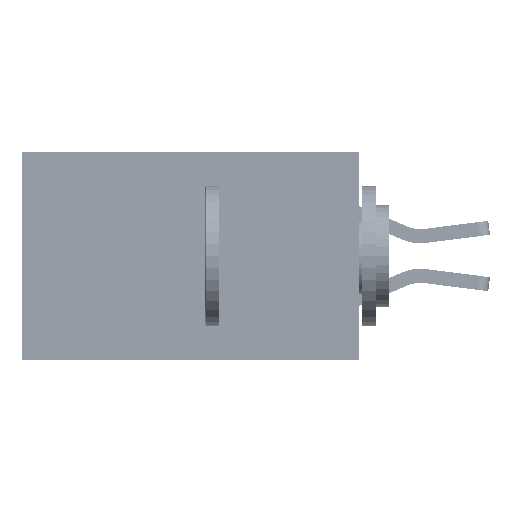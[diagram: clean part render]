
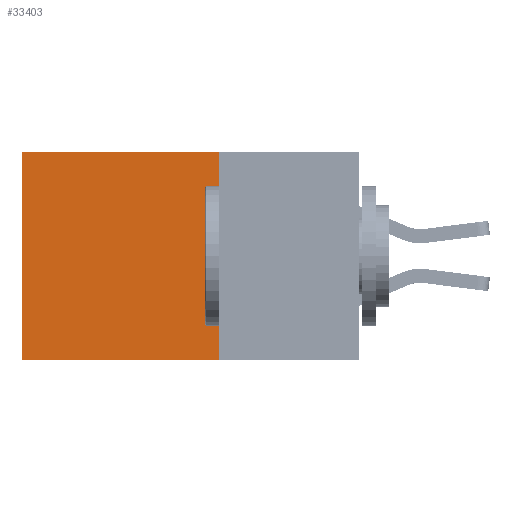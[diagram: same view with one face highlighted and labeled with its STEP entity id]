
A CAD part, left-side view. The second image highlights one B-rep face of the part: STEP entity #33403.
In plain terms, the highlighted planar face has unit normal (-1, 0, 0).
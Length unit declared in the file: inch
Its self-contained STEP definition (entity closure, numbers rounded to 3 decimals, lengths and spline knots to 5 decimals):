
#585 = VECTOR ( 'NONE', #14574, 39.37008 ) ;
#1162 = ORIENTED_EDGE ( 'NONE', *, *, #31129, .T. ) ;
#2350 = EDGE_CURVE ( 'NONE', #20033, #5243, #16051, .T. ) ;
#2531 = LINE ( 'NONE', #8172, #585 ) ;
#5243 = VERTEX_POINT ( 'NONE', #13102 ) ;
#6164 = VECTOR ( 'NONE', #26011, 39.37008 ) ;
#6791 = DIRECTION ( 'NONE',  ( 0., 0., -1. ) ) ;
#8172 = CARTESIAN_POINT ( 'NONE',  ( 0.2875, 0.25, -0.37 ) ) ;
#10236 = VERTEX_POINT ( 'NONE', #18625 ) ;
#10490 = DIRECTION ( 'NONE',  ( 0., 0., -1. ) ) ;
#10827 = ORIENTED_EDGE ( 'NONE', *, *, #2350, .F. ) ;
#13102 = CARTESIAN_POINT ( 'NONE',  ( 0.2875, 0.25, -0.37 ) ) ;
#13211 = PLANE ( 'NONE',  #18432 ) ;
#14574 = DIRECTION ( 'NONE',  ( 0., 1., 0. ) ) ;
#16051 = LINE ( 'NONE', #26485, #37288 ) ;
#18246 = CARTESIAN_POINT ( 'NONE',  ( 0.2875, 0.25, 0. ) ) ;
#18390 = EDGE_CURVE ( 'NONE', #5243, #10236, #2531, .T. ) ;
#18432 = AXIS2_PLACEMENT_3D ( 'NONE', #22139, #25239, #6791 ) ;
#18625 = CARTESIAN_POINT ( 'NONE',  ( 0.2875, 0.6, -0.37 ) ) ;
#20033 = VERTEX_POINT ( 'NONE', #18246 ) ;
#20118 = FACE_OUTER_BOUND ( 'NONE', #20454, .T. ) ;
#20174 = CARTESIAN_POINT ( 'NONE',  ( 0.2875, 0.6, 0. ) ) ;
#20454 = EDGE_LOOP ( 'NONE', ( #1162, #30225, #10827, #31787 ) ) ;
#20589 = LINE ( 'NONE', #32049, #6164 ) ;
#21209 = VERTEX_POINT ( 'NONE', #39591 ) ;
#22139 = CARTESIAN_POINT ( 'NONE',  ( 0.2875, 0.25, 0. ) ) ;
#25239 = DIRECTION ( 'NONE',  ( 1., 0., 0. ) ) ;
#25583 = LINE ( 'NONE', #20174, #37116 ) ;
#26011 = DIRECTION ( 'NONE',  ( 0., 1., 0. ) ) ;
#26485 = CARTESIAN_POINT ( 'NONE',  ( 0.2875, 0.25, 0. ) ) ;
#30225 = ORIENTED_EDGE ( 'NONE', *, *, #18390, .F. ) ;
#31129 = EDGE_CURVE ( 'NONE', #21209, #10236, #25583, .T. ) ;
#31787 = ORIENTED_EDGE ( 'NONE', *, *, #33432, .T. ) ;
#32049 = CARTESIAN_POINT ( 'NONE',  ( 0.2875, 0.25, 0. ) ) ;
#32804 = DIRECTION ( 'NONE',  ( 0., 0., -1. ) ) ;
#33403 = ADVANCED_FACE ( 'NONE', ( #20118 ), #13211, .F. ) ;
#33432 = EDGE_CURVE ( 'NONE', #20033, #21209, #20589, .T. ) ;
#37116 = VECTOR ( 'NONE', #10490, 39.37008 ) ;
#37288 = VECTOR ( 'NONE', #32804, 39.37008 ) ;
#39591 = CARTESIAN_POINT ( 'NONE',  ( 0.2875, 0.6, 0. ) ) ;
